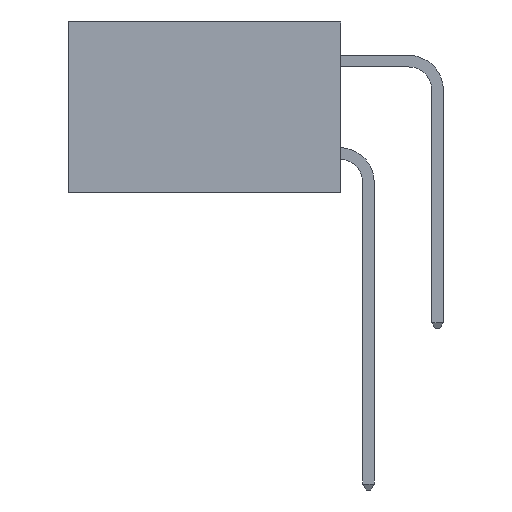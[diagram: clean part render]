
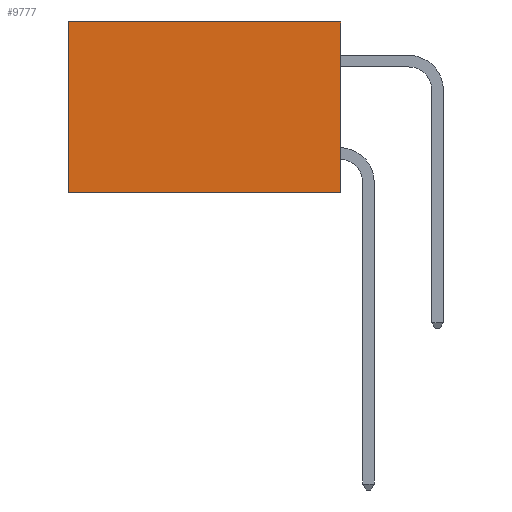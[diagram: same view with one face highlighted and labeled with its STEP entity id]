
A CAD part, left-side view. The second image highlights one B-rep face of the part: STEP entity #9777.
In plain terms, the highlighted planar face has unit normal (-1, 0, 0).
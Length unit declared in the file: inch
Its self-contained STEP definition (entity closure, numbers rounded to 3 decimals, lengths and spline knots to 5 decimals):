
#535 = LINE ( 'NONE', #2580, #4360 ) ;
#681 = VECTOR ( 'NONE', #7760, 39.37008 ) ;
#1054 = VERTEX_POINT ( 'NONE', #11522 ) ;
#2053 = VERTEX_POINT ( 'NONE', #6558 ) ;
#2540 = DIRECTION ( 'NONE',  ( 0., 0., -1. ) ) ;
#2580 = CARTESIAN_POINT ( 'NONE',  ( 0.277, 0.59, -0.37 ) ) ;
#2691 = LINE ( 'NONE', #9873, #5133 ) ;
#2983 = PLANE ( 'NONE',  #6055 ) ;
#4300 = ORIENTED_EDGE ( 'NONE', *, *, #5892, .T. ) ;
#4360 = VECTOR ( 'NONE', #2540, 39.37008 ) ;
#4529 = EDGE_CURVE ( 'NONE', #2053, #1054, #8868, .T. ) ;
#5133 = VECTOR ( 'NONE', #9708, 39.37008 ) ;
#5299 = CARTESIAN_POINT ( 'NONE',  ( 0.277, 0.59, 0. ) ) ;
#5406 = DIRECTION ( 'NONE',  ( 0., 0., -1. ) ) ;
#5664 = EDGE_CURVE ( 'NONE', #1054, #9817, #2691, .T. ) ;
#5748 = EDGE_LOOP ( 'NONE', ( #8374, #10956, #11840, #4300 ) ) ;
#5892 = EDGE_CURVE ( 'NONE', #2053, #5988, #10198, .T. ) ;
#5988 = VERTEX_POINT ( 'NONE', #5299 ) ;
#5992 = DIRECTION ( 'NONE',  ( 1., 0., 0. ) ) ;
#6020 = CARTESIAN_POINT ( 'NONE',  ( 0.277, 0., -0.37 ) ) ;
#6055 = AXIS2_PLACEMENT_3D ( 'NONE', #6020, #5992, #5406 ) ;
#6273 = CARTESIAN_POINT ( 'NONE',  ( 0.277, 0., 0. ) ) ;
#6558 = CARTESIAN_POINT ( 'NONE',  ( 0.277, 0., 0. ) ) ;
#6608 = FACE_OUTER_BOUND ( 'NONE', #5748, .T. ) ;
#6767 = DIRECTION ( 'NONE',  ( 0., 1., 0. ) ) ;
#7731 = CARTESIAN_POINT ( 'NONE',  ( 0.277, 0., -0.37 ) ) ;
#7760 = DIRECTION ( 'NONE',  ( 0., 0., -1. ) ) ;
#8374 = ORIENTED_EDGE ( 'NONE', *, *, #9629, .T. ) ;
#8868 = LINE ( 'NONE', #7731, #681 ) ;
#9036 = CARTESIAN_POINT ( 'NONE',  ( 0.277, 0.59, -0.37 ) ) ;
#9629 = EDGE_CURVE ( 'NONE', #5988, #9817, #535, .T. ) ;
#9708 = DIRECTION ( 'NONE',  ( 0., 1., 0. ) ) ;
#9777 = ADVANCED_FACE ( 'NONE', ( #6608 ), #2983, .F. ) ;
#9817 = VERTEX_POINT ( 'NONE', #9036 ) ;
#9873 = CARTESIAN_POINT ( 'NONE',  ( 0.277, 0., -0.37 ) ) ;
#10198 = LINE ( 'NONE', #6273, #10801 ) ;
#10801 = VECTOR ( 'NONE', #6767, 39.37008 ) ;
#10956 = ORIENTED_EDGE ( 'NONE', *, *, #5664, .F. ) ;
#11522 = CARTESIAN_POINT ( 'NONE',  ( 0.277, 0., -0.37 ) ) ;
#11840 = ORIENTED_EDGE ( 'NONE', *, *, #4529, .F. ) ;
